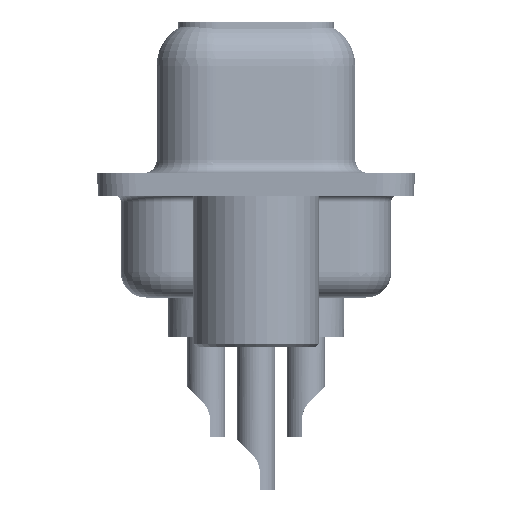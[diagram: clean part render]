
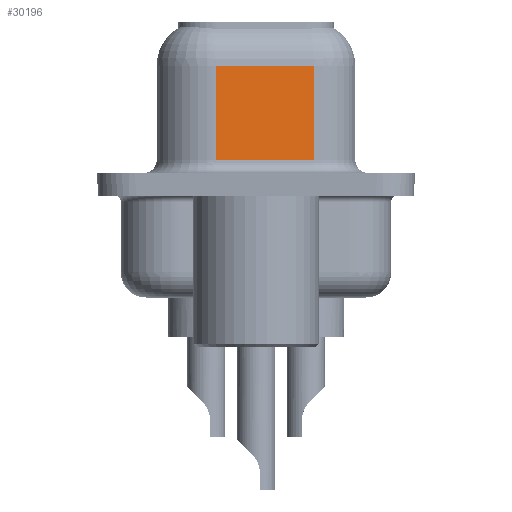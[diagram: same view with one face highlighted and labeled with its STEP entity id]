
A CAD part, left-side view. The second image highlights one B-rep face of the part: STEP entity #30196.
In plain terms, the highlighted planar face has unit normal (-0.985, -0.174, 0).
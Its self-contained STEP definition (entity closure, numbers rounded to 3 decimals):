
#178 = EDGE_CURVE ( 'NONE', #3091, #19227, #27717, .T. ) ;
#239 = VERTEX_POINT ( 'NONE', #31470 ) ;
#415 = DIRECTION ( 'NONE',  ( 0.985, 0.174, 0. ) ) ;
#1045 = CARTESIAN_POINT ( 'NONE',  ( 5.068, -2.297, 4.7 ) ) ;
#1512 = EDGE_LOOP ( 'NONE', ( #12791, #16913, #32463, #3309 ) ) ;
#3091 = VERTEX_POINT ( 'NONE', #14186 ) ;
#3309 = ORIENTED_EDGE ( 'NONE', *, *, #178, .T. ) ;
#6661 = DIRECTION ( 'NONE',  ( 0., 0., -1. ) ) ;
#7053 = CARTESIAN_POINT ( 'NONE',  ( 5.068, -2.297, 0.95 ) ) ;
#7109 = CARTESIAN_POINT ( 'NONE',  ( 4.38, 1.603, 6.45 ) ) ;
#7299 = FACE_OUTER_BOUND ( 'NONE', #1512, .T. ) ;
#7980 = EDGE_CURVE ( 'NONE', #239, #32764, #31480, .T. ) ;
#9499 = LINE ( 'NONE', #33245, #11337 ) ;
#11337 = VECTOR ( 'NONE', #27031, 1000. ) ;
#12791 = ORIENTED_EDGE ( 'NONE', *, *, #24053, .F. ) ;
#13305 = PLANE ( 'NONE',  #43457 ) ;
#14186 = CARTESIAN_POINT ( 'NONE',  ( 4.38, 1.603, 0.95 ) ) ;
#14598 = DIRECTION ( 'NONE',  ( -0.174, 0.985, 0. ) ) ;
#16913 = ORIENTED_EDGE ( 'NONE', *, *, #7980, .T. ) ;
#19227 = VERTEX_POINT ( 'NONE', #21962 ) ;
#21298 = VECTOR ( 'NONE', #14598, 1000. ) ;
#21464 = CARTESIAN_POINT ( 'NONE',  ( 4.38, 1.603, 4.7 ) ) ;
#21962 = CARTESIAN_POINT ( 'NONE',  ( 5.068, -2.297, 0.95 ) ) ;
#23785 = LINE ( 'NONE', #7109, #43038 ) ;
#24053 = EDGE_CURVE ( 'NONE', #239, #19227, #9499, .T. ) ;
#26851 = DIRECTION ( 'NONE',  ( -0.174, 0.985, 0. ) ) ;
#27031 = DIRECTION ( 'NONE',  ( 0., 0., -1. ) ) ;
#27717 = LINE ( 'NONE', #7053, #41034 ) ;
#30196 = ADVANCED_FACE ( 'NONE', ( #7299 ), #13305, .F. ) ;
#30636 = CARTESIAN_POINT ( 'NONE',  ( 5.068, -2.297, 6.45 ) ) ;
#31470 = CARTESIAN_POINT ( 'NONE',  ( 5.068, -2.297, 4.7 ) ) ;
#31480 = LINE ( 'NONE', #1045, #21298 ) ;
#32463 = ORIENTED_EDGE ( 'NONE', *, *, #35292, .T. ) ;
#32764 = VERTEX_POINT ( 'NONE', #21464 ) ;
#33245 = CARTESIAN_POINT ( 'NONE',  ( 5.068, -2.297, 6.45 ) ) ;
#35292 = EDGE_CURVE ( 'NONE', #32764, #3091, #23785, .T. ) ;
#41029 = DIRECTION ( 'NONE',  ( 0.174, -0.985, 0. ) ) ;
#41034 = VECTOR ( 'NONE', #41029, 1000. ) ;
#43038 = VECTOR ( 'NONE', #6661, 1000. ) ;
#43457 = AXIS2_PLACEMENT_3D ( 'NONE', #30636, #415, #26851 ) ;
